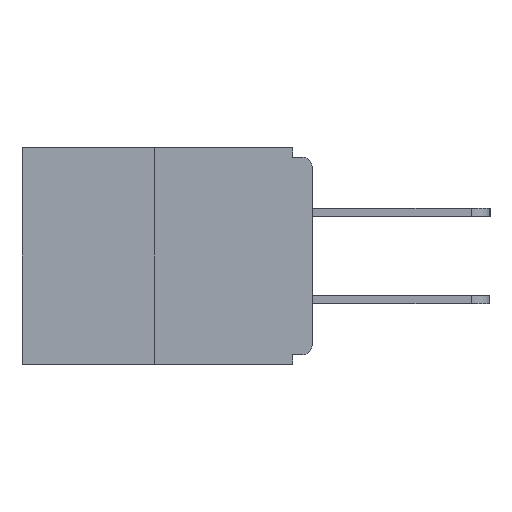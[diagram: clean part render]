
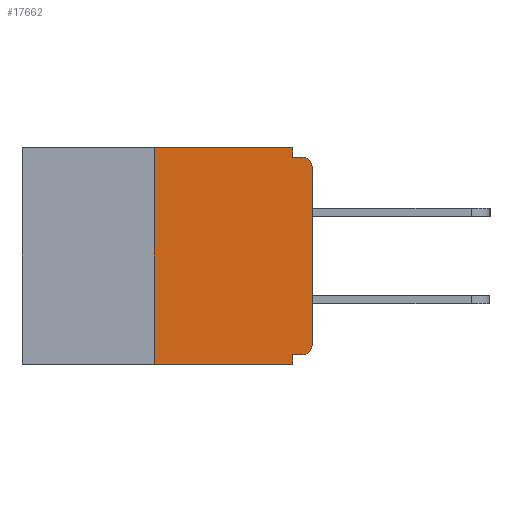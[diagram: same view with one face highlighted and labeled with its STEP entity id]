
A CAD part, left-side view. The second image highlights one B-rep face of the part: STEP entity #17662.
In plain terms, the highlighted planar face has unit normal (-1, 0, 0).
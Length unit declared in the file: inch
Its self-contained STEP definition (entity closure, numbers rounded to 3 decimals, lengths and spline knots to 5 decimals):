
#254 = CARTESIAN_POINT ( 'NONE',  ( 0., 0.031, -0.343 ) ) ;
#357 = ORIENTED_EDGE ( 'NONE', *, *, #11358, .F. ) ;
#521 = VERTEX_POINT ( 'NONE', #12599 ) ;
#924 = VECTOR ( 'NONE', #7941, 39.37008 ) ;
#1417 = AXIS2_PLACEMENT_3D ( 'NONE', #12337, #10887, #2718 ) ;
#1532 = ORIENTED_EDGE ( 'NONE', *, *, #3823, .F. ) ;
#1584 = CARTESIAN_POINT ( 'NONE',  ( 0., 0.015, -0.015 ) ) ;
#1634 = CARTESIAN_POINT ( 'NONE',  ( 0., 0.031, 0. ) ) ;
#2450 = DIRECTION ( 'NONE',  ( 0., 0., -1. ) ) ;
#2457 = CARTESIAN_POINT ( 'NONE',  ( 0., 0.46, 0. ) ) ;
#2503 = EDGE_CURVE ( 'NONE', #10659, #17180, #8624, .T. ) ;
#2550 = LINE ( 'NONE', #1634, #17858 ) ;
#2718 = DIRECTION ( 'NONE',  ( 0., 0., -1. ) ) ;
#3048 = CARTESIAN_POINT ( 'NONE',  ( 0., 0., -0.015 ) ) ;
#3225 = CARTESIAN_POINT ( 'NONE',  ( 0., 0.031, -0.328 ) ) ;
#3514 = CARTESIAN_POINT ( 'NONE',  ( 0., 0.015, -0.328 ) ) ;
#3564 = ORIENTED_EDGE ( 'NONE', *, *, #13788, .F. ) ;
#3716 = CARTESIAN_POINT ( 'NONE',  ( 0., 0.031, 0. ) ) ;
#3819 = VERTEX_POINT ( 'NONE', #5692 ) ;
#3823 = EDGE_CURVE ( 'NONE', #5419, #521, #2550, .T. ) ;
#5220 = CARTESIAN_POINT ( 'NONE',  ( 0., 0., -0.313 ) ) ;
#5258 = DIRECTION ( 'NONE',  ( 1., 0., 0. ) ) ;
#5343 = DIRECTION ( 'NONE',  ( 0., 0., 1. ) ) ;
#5419 = VERTEX_POINT ( 'NONE', #3716 ) ;
#5549 = DIRECTION ( 'NONE',  ( 0., -1., 0. ) ) ;
#5652 = VECTOR ( 'NONE', #5973, 39.37008 ) ;
#5692 = CARTESIAN_POINT ( 'NONE',  ( 0., 0.25, 0. ) ) ;
#5860 = ORIENTED_EDGE ( 'NONE', *, *, #7503, .F. ) ;
#5911 = ORIENTED_EDGE ( 'NONE', *, *, #7977, .T. ) ;
#5952 = CARTESIAN_POINT ( 'NONE',  ( 0., 0.25, -0.343 ) ) ;
#5973 = DIRECTION ( 'NONE',  ( 0., -1., 0. ) ) ;
#7503 = EDGE_CURVE ( 'NONE', #3819, #5419, #16694, .T. ) ;
#7561 = VECTOR ( 'NONE', #15634, 39.37008 ) ;
#7682 = EDGE_CURVE ( 'NONE', #17180, #11159, #15368, .T. ) ;
#7724 = EDGE_CURVE ( 'NONE', #521, #13006, #14287, .T. ) ;
#7840 = VERTEX_POINT ( 'NONE', #5952 ) ;
#7941 = DIRECTION ( 'NONE',  ( 0., -1., 0. ) ) ;
#7977 = EDGE_CURVE ( 'NONE', #7840, #15988, #11722, .T. ) ;
#8624 = CIRCLE ( 'NONE', #15688, 0.015 ) ;
#8849 = VECTOR ( 'NONE', #5343, 39.37008 ) ;
#9070 = EDGE_CURVE ( 'NONE', #12184, #15988, #13812, .T. ) ;
#9270 = LINE ( 'NONE', #16337, #8849 ) ;
#9394 = ORIENTED_EDGE ( 'NONE', *, *, #9070, .F. ) ;
#10316 = DIRECTION ( 'NONE',  ( -1., 0., 0. ) ) ;
#10659 = VERTEX_POINT ( 'NONE', #3514 ) ;
#10887 = DIRECTION ( 'NONE',  ( -1., 0., 0. ) ) ;
#10972 = EDGE_CURVE ( 'NONE', #11159, #13006, #13370, .T. ) ;
#10990 = AXIS2_PLACEMENT_3D ( 'NONE', #2457, #5258, #14896 ) ;
#11102 = VECTOR ( 'NONE', #5549, 39.37008 ) ;
#11159 = VERTEX_POINT ( 'NONE', #12985 ) ;
#11241 = DIRECTION ( 'NONE',  ( 0., 0., -1. ) ) ;
#11358 = EDGE_CURVE ( 'NONE', #10659, #12184, #15584, .T. ) ;
#11722 = LINE ( 'NONE', #13525, #924 ) ;
#11803 = ORIENTED_EDGE ( 'NONE', *, *, #7682, .T. ) ;
#11843 = DIRECTION ( 'NONE',  ( 0., 0., -1. ) ) ;
#11968 = CARTESIAN_POINT ( 'NONE',  ( 0., 0., -0.328 ) ) ;
#11984 = ORIENTED_EDGE ( 'NONE', *, *, #2503, .T. ) ;
#12184 = VERTEX_POINT ( 'NONE', #3225 ) ;
#12337 = CARTESIAN_POINT ( 'NONE',  ( 0., 0.015, -0.03 ) ) ;
#12599 = CARTESIAN_POINT ( 'NONE',  ( 0., 0.031, -0.015 ) ) ;
#12985 = CARTESIAN_POINT ( 'NONE',  ( 0., 0., -0.03 ) ) ;
#13006 = VERTEX_POINT ( 'NONE', #1584 ) ;
#13370 = CIRCLE ( 'NONE', #1417, 0.015 ) ;
#13525 = CARTESIAN_POINT ( 'NONE',  ( 0., 0.46, -0.343 ) ) ;
#13788 = EDGE_CURVE ( 'NONE', #7840, #3819, #9270, .T. ) ;
#13812 = LINE ( 'NONE', #17547, #17078 ) ;
#14196 = FACE_OUTER_BOUND ( 'NONE', #15393, .T. ) ;
#14287 = LINE ( 'NONE', #3048, #5652 ) ;
#14896 = DIRECTION ( 'NONE',  ( 0., 0., -1. ) ) ;
#15124 = CARTESIAN_POINT ( 'NONE',  ( 0., 0.46, 0. ) ) ;
#15368 = LINE ( 'NONE', #15396, #7561 ) ;
#15393 = EDGE_LOOP ( 'NONE', ( #5860, #3564, #5911, #9394, #357, #11984, #11803, #16467, #15959, #1532 ) ) ;
#15396 = CARTESIAN_POINT ( 'NONE',  ( 0., 0., 0. ) ) ;
#15584 = LINE ( 'NONE', #11968, #17328 ) ;
#15634 = DIRECTION ( 'NONE',  ( 0., 0., 1. ) ) ;
#15688 = AXIS2_PLACEMENT_3D ( 'NONE', #17185, #10316, #2450 ) ;
#15959 = ORIENTED_EDGE ( 'NONE', *, *, #7724, .F. ) ;
#15988 = VERTEX_POINT ( 'NONE', #254 ) ;
#16212 = DIRECTION ( 'NONE',  ( 0., 1., 0. ) ) ;
#16337 = CARTESIAN_POINT ( 'NONE',  ( 0., 0.25, 0. ) ) ;
#16467 = ORIENTED_EDGE ( 'NONE', *, *, #10972, .T. ) ;
#16694 = LINE ( 'NONE', #15124, #11102 ) ;
#17078 = VECTOR ( 'NONE', #11843, 39.37008 ) ;
#17180 = VERTEX_POINT ( 'NONE', #5220 ) ;
#17185 = CARTESIAN_POINT ( 'NONE',  ( 0., 0.015, -0.313 ) ) ;
#17328 = VECTOR ( 'NONE', #16212, 39.37008 ) ;
#17547 = CARTESIAN_POINT ( 'NONE',  ( 0., 0.031, -0.343 ) ) ;
#17595 = PLANE ( 'NONE',  #10990 ) ;
#17662 = ADVANCED_FACE ( 'NONE', ( #14196 ), #17595, .F. ) ;
#17858 = VECTOR ( 'NONE', #11241, 39.37008 ) ;
